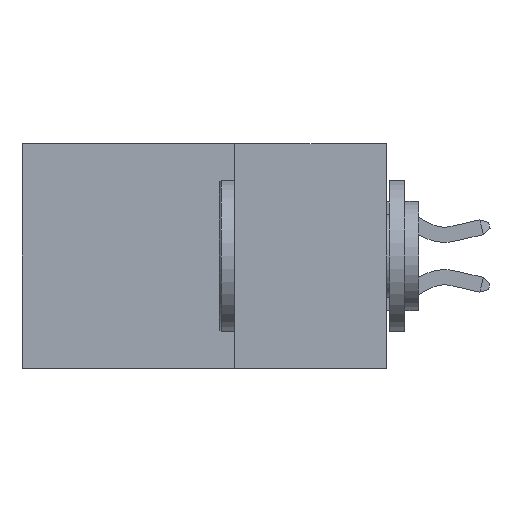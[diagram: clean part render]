
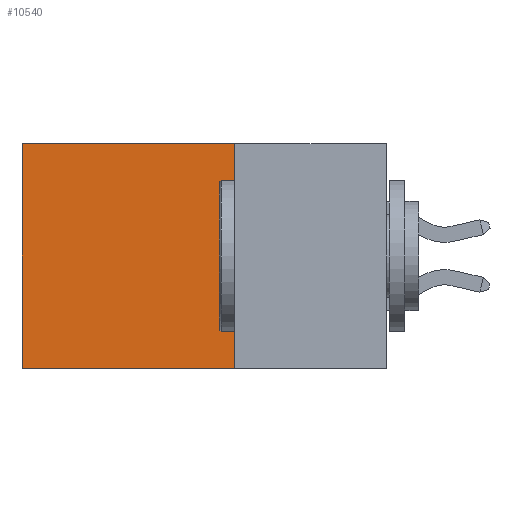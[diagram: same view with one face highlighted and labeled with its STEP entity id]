
A CAD part, left-side view. The second image highlights one B-rep face of the part: STEP entity #10540.
In plain terms, the highlighted planar face has unit normal (-1, 0, 0).
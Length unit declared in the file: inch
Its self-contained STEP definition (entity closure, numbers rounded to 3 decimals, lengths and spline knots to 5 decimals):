
#1322 = VERTEX_POINT ( 'NONE', #30165 ) ;
#1796 = DIRECTION ( 'NONE',  ( 0., 0., -1. ) ) ;
#3052 = EDGE_LOOP ( 'NONE', ( #30390, #25678, #15590, #28026 ) ) ;
#4061 = FACE_OUTER_BOUND ( 'NONE', #3052, .T. ) ;
#4553 = EDGE_CURVE ( 'NONE', #1322, #11932, #10298, .T. ) ;
#6815 = VECTOR ( 'NONE', #31393, 39.37008 ) ;
#7552 = VERTEX_POINT ( 'NONE', #18863 ) ;
#9203 = DIRECTION ( 'NONE',  ( 0., 0., -1. ) ) ;
#9893 = CARTESIAN_POINT ( 'NONE',  ( 0.298, 0.6, 0. ) ) ;
#10298 = LINE ( 'NONE', #26324, #22480 ) ;
#10540 = ADVANCED_FACE ( 'NONE', ( #4061 ), #14164, .F. ) ;
#11316 = CARTESIAN_POINT ( 'NONE',  ( 0.298, 0.25, 0. ) ) ;
#11581 = EDGE_CURVE ( 'NONE', #7552, #13852, #11741, .T. ) ;
#11741 = LINE ( 'NONE', #11316, #23135 ) ;
#11932 = VERTEX_POINT ( 'NONE', #24533 ) ;
#13852 = VERTEX_POINT ( 'NONE', #9893 ) ;
#14093 = CARTESIAN_POINT ( 'NONE',  ( 0.298, 0.6, 0. ) ) ;
#14164 = PLANE ( 'NONE',  #14510 ) ;
#14177 = LINE ( 'NONE', #17074, #6815 ) ;
#14510 = AXIS2_PLACEMENT_3D ( 'NONE', #30919, #16608, #1796 ) ;
#15551 = EDGE_CURVE ( 'NONE', #7552, #1322, #14177, .T. ) ;
#15590 = ORIENTED_EDGE ( 'NONE', *, *, #15551, .F. ) ;
#16608 = DIRECTION ( 'NONE',  ( 1., 0., 0. ) ) ;
#17074 = CARTESIAN_POINT ( 'NONE',  ( 0.298, 0.25, 0. ) ) ;
#18863 = CARTESIAN_POINT ( 'NONE',  ( 0.298, 0.25, 0. ) ) ;
#22480 = VECTOR ( 'NONE', #26210, 39.37008 ) ;
#23135 = VECTOR ( 'NONE', #28233, 39.37008 ) ;
#23637 = VECTOR ( 'NONE', #9203, 39.37008 ) ;
#24385 = LINE ( 'NONE', #14093, #23637 ) ;
#24533 = CARTESIAN_POINT ( 'NONE',  ( 0.298, 0.6, -0.37 ) ) ;
#25678 = ORIENTED_EDGE ( 'NONE', *, *, #4553, .F. ) ;
#26210 = DIRECTION ( 'NONE',  ( 0., 1., 0. ) ) ;
#26324 = CARTESIAN_POINT ( 'NONE',  ( 0.298, 0.25, -0.37 ) ) ;
#28026 = ORIENTED_EDGE ( 'NONE', *, *, #11581, .T. ) ;
#28233 = DIRECTION ( 'NONE',  ( 0., 1., 0. ) ) ;
#29418 = EDGE_CURVE ( 'NONE', #13852, #11932, #24385, .T. ) ;
#30165 = CARTESIAN_POINT ( 'NONE',  ( 0.298, 0.25, -0.37 ) ) ;
#30390 = ORIENTED_EDGE ( 'NONE', *, *, #29418, .T. ) ;
#30919 = CARTESIAN_POINT ( 'NONE',  ( 0.298, 0.25, 0. ) ) ;
#31393 = DIRECTION ( 'NONE',  ( 0., 0., -1. ) ) ;
